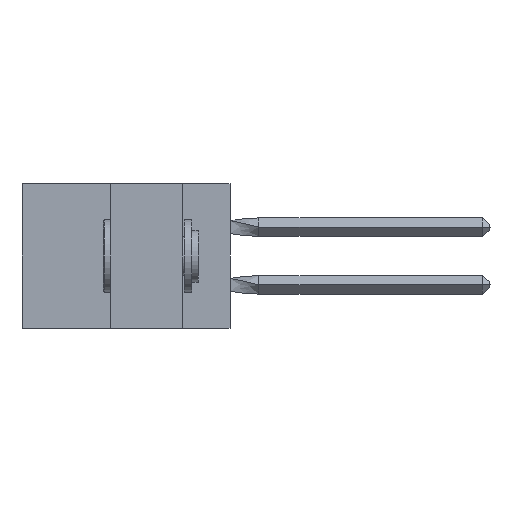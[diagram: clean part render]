
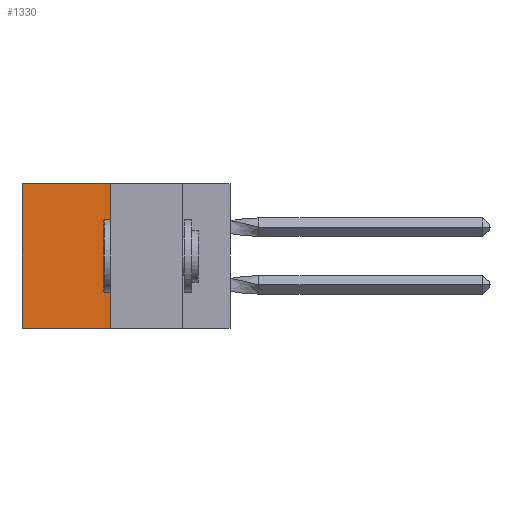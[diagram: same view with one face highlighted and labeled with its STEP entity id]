
A CAD part, left-side view. The second image highlights one B-rep face of the part: STEP entity #1330.
In plain terms, the highlighted planar face has unit normal (-1, 0, 0).
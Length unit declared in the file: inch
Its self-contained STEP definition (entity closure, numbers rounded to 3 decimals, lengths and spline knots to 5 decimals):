
#965 = CARTESIAN_POINT ( 'NONE',  ( 0.305, 0.413, -0.5 ) ) ;
#1015 = VECTOR ( 'NONE', #40184, 39.37008 ) ;
#1330 = ADVANCED_FACE ( 'NONE', ( #27103 ), #6983, .F. ) ;
#1542 = VERTEX_POINT ( 'NONE', #34839 ) ;
#1811 = ORIENTED_EDGE ( 'NONE', *, *, #7844, .T. ) ;
#2216 = CARTESIAN_POINT ( 'NONE',  ( 0.305, 0.413, 0. ) ) ;
#3298 = EDGE_CURVE ( 'NONE', #39055, #1542, #10607, .T. ) ;
#3350 = LINE ( 'NONE', #16647, #38679 ) ;
#4030 = DIRECTION ( 'NONE',  ( 0., 0., -1. ) ) ;
#4962 = CARTESIAN_POINT ( 'NONE',  ( 0.305, 0.413, -0.5 ) ) ;
#6418 = EDGE_LOOP ( 'NONE', ( #11123, #16451, #33872, #1811 ) ) ;
#6983 = PLANE ( 'NONE',  #14208 ) ;
#7176 = VECTOR ( 'NONE', #27681, 39.37008 ) ;
#7256 = CARTESIAN_POINT ( 'NONE',  ( 0.305, 0.413, -0.5 ) ) ;
#7844 = EDGE_CURVE ( 'NONE', #18048, #11309, #12178, .T. ) ;
#9701 = EDGE_CURVE ( 'NONE', #18048, #39055, #24139, .T. ) ;
#10607 = LINE ( 'NONE', #23898, #1015 ) ;
#11123 = ORIENTED_EDGE ( 'NONE', *, *, #27337, .T. ) ;
#11309 = VERTEX_POINT ( 'NONE', #26526 ) ;
#12178 = LINE ( 'NONE', #14438, #7176 ) ;
#14208 = AXIS2_PLACEMENT_3D ( 'NONE', #7256, #20192, #29496 ) ;
#14438 = CARTESIAN_POINT ( 'NONE',  ( 0.305, 0.413, 0. ) ) ;
#16451 = ORIENTED_EDGE ( 'NONE', *, *, #3298, .F. ) ;
#16647 = CARTESIAN_POINT ( 'NONE',  ( 0.305, 0.72, -0.5 ) ) ;
#18048 = VERTEX_POINT ( 'NONE', #2216 ) ;
#20192 = DIRECTION ( 'NONE',  ( 1., 0., 0. ) ) ;
#23898 = CARTESIAN_POINT ( 'NONE',  ( 0.305, 0.413, -0.5 ) ) ;
#24139 = LINE ( 'NONE', #965, #31210 ) ;
#26526 = CARTESIAN_POINT ( 'NONE',  ( 0.305, 0.72, 0. ) ) ;
#27103 = FACE_OUTER_BOUND ( 'NONE', #6418, .T. ) ;
#27337 = EDGE_CURVE ( 'NONE', #11309, #1542, #3350, .T. ) ;
#27681 = DIRECTION ( 'NONE',  ( 0., 1., 0. ) ) ;
#29496 = DIRECTION ( 'NONE',  ( 0., 0., -1. ) ) ;
#31210 = VECTOR ( 'NONE', #34119, 39.37008 ) ;
#33872 = ORIENTED_EDGE ( 'NONE', *, *, #9701, .F. ) ;
#34119 = DIRECTION ( 'NONE',  ( 0., 0., -1. ) ) ;
#34839 = CARTESIAN_POINT ( 'NONE',  ( 0.305, 0.72, -0.5 ) ) ;
#38679 = VECTOR ( 'NONE', #4030, 39.37008 ) ;
#39055 = VERTEX_POINT ( 'NONE', #4962 ) ;
#40184 = DIRECTION ( 'NONE',  ( 0., 1., 0. ) ) ;
